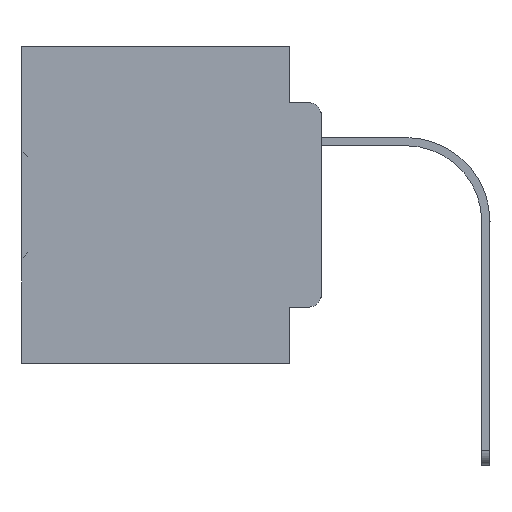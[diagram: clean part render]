
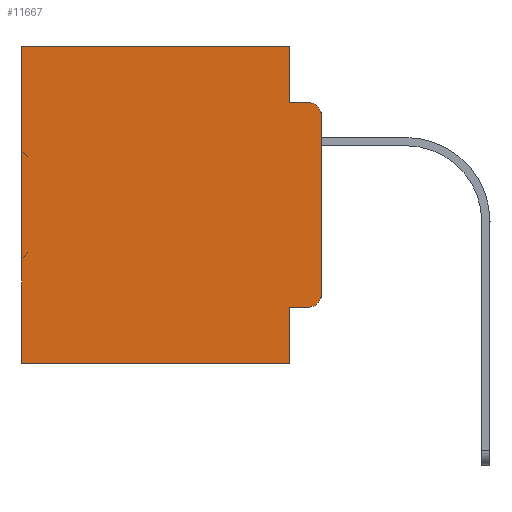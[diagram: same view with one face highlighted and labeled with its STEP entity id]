
A CAD part, left-side view. The second image highlights one B-rep face of the part: STEP entity #11667.
In plain terms, the highlighted planar face has unit normal (-1, 0, 0).
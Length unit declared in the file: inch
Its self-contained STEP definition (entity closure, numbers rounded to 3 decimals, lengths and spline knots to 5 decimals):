
#683 = VERTEX_POINT ( 'NONE', #31722 ) ;
#864 = CARTESIAN_POINT ( 'NONE',  ( 0.298, 0.02, -0.0885 ) ) ;
#2679 = DIRECTION ( 'NONE',  ( 0., 0., -1. ) ) ;
#2912 = DIRECTION ( 'NONE',  ( 0., 0., -1. ) ) ;
#5111 = VERTEX_POINT ( 'NONE', #15395 ) ;
#5186 = ORIENTED_EDGE ( 'NONE', *, *, #19873, .F. ) ;
#6548 = ORIENTED_EDGE ( 'NONE', *, *, #14699, .F. ) ;
#7915 = VECTOR ( 'NONE', #10473, 39.37008 ) ;
#8126 = CARTESIAN_POINT ( 'NONE',  ( 0.298, 0.051, 0. ) ) ;
#8137 = LINE ( 'NONE', #22855, #13507 ) ;
#8353 = LINE ( 'NONE', #14416, #17982 ) ;
#8695 = DIRECTION ( 'NONE',  ( 0., -1., 0. ) ) ;
#9843 = AXIS2_PLACEMENT_3D ( 'NONE', #10184, #36247, #30550 ) ;
#10184 = CARTESIAN_POINT ( 'NONE',  ( 0.298, 0.02, -0.3915 ) ) ;
#10473 = DIRECTION ( 'NONE',  ( 0., 0., -1. ) ) ;
#10853 = CARTESIAN_POINT ( 'NONE',  ( 0.298, 0., 0. ) ) ;
#10874 = ORIENTED_EDGE ( 'NONE', *, *, #19233, .T. ) ;
#11622 = ORIENTED_EDGE ( 'NONE', *, *, #29310, .F. ) ;
#11667 = ADVANCED_FACE ( 'NONE', ( #33702 ), #21825, .F. ) ;
#11980 = EDGE_CURVE ( 'NONE', #24811, #5111, #13129, .T. ) ;
#13129 = LINE ( 'NONE', #30475, #7915 ) ;
#13137 = CARTESIAN_POINT ( 'NONE',  ( 0.298, 0., 0. ) ) ;
#13507 = VECTOR ( 'NONE', #8695, 39.37008 ) ;
#14056 = DIRECTION ( 'NONE',  ( 0., 0., -1. ) ) ;
#14416 = CARTESIAN_POINT ( 'NONE',  ( 0.298, 0.051, -0.4115 ) ) ;
#14699 = EDGE_CURVE ( 'NONE', #35390, #24124, #34506, .T. ) ;
#15132 = VECTOR ( 'NONE', #25929, 39.37008 ) ;
#15395 = CARTESIAN_POINT ( 'NONE',  ( 0.298, 0.051, -0.0885 ) ) ;
#15491 = ORIENTED_EDGE ( 'NONE', *, *, #23393, .T. ) ;
#15737 = AXIS2_PLACEMENT_3D ( 'NONE', #13137, #30297, #16359 ) ;
#15740 = LINE ( 'NONE', #35930, #32511 ) ;
#15836 = EDGE_CURVE ( 'NONE', #32039, #35390, #34621, .T. ) ;
#16308 = VERTEX_POINT ( 'NONE', #29089 ) ;
#16359 = DIRECTION ( 'NONE',  ( 0., 0., -1. ) ) ;
#16947 = CARTESIAN_POINT ( 'NONE',  ( 0.298, 0.02, -0.1085 ) ) ;
#17837 = LINE ( 'NONE', #34813, #15132 ) ;
#17982 = VECTOR ( 'NONE', #25519, 39.37008 ) ;
#18398 = CIRCLE ( 'NONE', #24407, 0.02 ) ;
#19233 = EDGE_CURVE ( 'NONE', #32039, #26867, #8353, .T. ) ;
#19412 = CARTESIAN_POINT ( 'NONE',  ( 0.298, 0.473, -0.5 ) ) ;
#19534 = ORIENTED_EDGE ( 'NONE', *, *, #30064, .T. ) ;
#19577 = VECTOR ( 'NONE', #2912, 39.37008 ) ;
#19873 = EDGE_CURVE ( 'NONE', #16308, #683, #36717, .T. ) ;
#20546 = EDGE_CURVE ( 'NONE', #23524, #24124, #15740, .T. ) ;
#21825 = PLANE ( 'NONE',  #15737 ) ;
#22612 = CARTESIAN_POINT ( 'NONE',  ( 0.298, 0., -0.5 ) ) ;
#22855 = CARTESIAN_POINT ( 'NONE',  ( 0.298, 0.051, -0.0885 ) ) ;
#23393 = EDGE_CURVE ( 'NONE', #24811, #23524, #17837, .T. ) ;
#23473 = CARTESIAN_POINT ( 'NONE',  ( 0.298, 0.051, 0. ) ) ;
#23524 = VERTEX_POINT ( 'NONE', #27598 ) ;
#24039 = ORIENTED_EDGE ( 'NONE', *, *, #11980, .F. ) ;
#24124 = VERTEX_POINT ( 'NONE', #19412 ) ;
#24407 = AXIS2_PLACEMENT_3D ( 'NONE', #16947, #36937, #25774 ) ;
#24553 = CARTESIAN_POINT ( 'NONE',  ( 0.298, 0.051, -0.4115 ) ) ;
#24631 = ORIENTED_EDGE ( 'NONE', *, *, #20546, .T. ) ;
#24811 = VERTEX_POINT ( 'NONE', #8126 ) ;
#25519 = DIRECTION ( 'NONE',  ( 0., -1., 0. ) ) ;
#25774 = DIRECTION ( 'NONE',  ( 0., 0., -1. ) ) ;
#25929 = DIRECTION ( 'NONE',  ( 0., 1., 0. ) ) ;
#26867 = VERTEX_POINT ( 'NONE', #27853 ) ;
#27598 = CARTESIAN_POINT ( 'NONE',  ( 0.298, 0.473, 0. ) ) ;
#27853 = CARTESIAN_POINT ( 'NONE',  ( 0.298, 0.02, -0.4115 ) ) ;
#27895 = ORIENTED_EDGE ( 'NONE', *, *, #28330, .T. ) ;
#28330 = EDGE_CURVE ( 'NONE', #26867, #683, #35167, .T. ) ;
#29089 = CARTESIAN_POINT ( 'NONE',  ( 0.298, 0., -0.1085 ) ) ;
#29310 = EDGE_CURVE ( 'NONE', #5111, #36928, #8137, .T. ) ;
#30064 = EDGE_CURVE ( 'NONE', #16308, #36928, #18398, .T. ) ;
#30297 = DIRECTION ( 'NONE',  ( 1., 0., 0. ) ) ;
#30400 = VECTOR ( 'NONE', #33943, 39.37008 ) ;
#30475 = CARTESIAN_POINT ( 'NONE',  ( 0.298, 0.051, 0. ) ) ;
#30550 = DIRECTION ( 'NONE',  ( 0., 0., -1. ) ) ;
#31722 = CARTESIAN_POINT ( 'NONE',  ( 0.298, 0., -0.3915 ) ) ;
#32039 = VERTEX_POINT ( 'NONE', #24553 ) ;
#32073 = ORIENTED_EDGE ( 'NONE', *, *, #15836, .F. ) ;
#32511 = VECTOR ( 'NONE', #2679, 39.37008 ) ;
#33051 = VECTOR ( 'NONE', #14056, 39.37008 ) ;
#33536 = CARTESIAN_POINT ( 'NONE',  ( 0.298, 0.051, -0.5 ) ) ;
#33702 = FACE_OUTER_BOUND ( 'NONE', #36355, .T. ) ;
#33943 = DIRECTION ( 'NONE',  ( 0., 1., 0. ) ) ;
#34506 = LINE ( 'NONE', #22612, #30400 ) ;
#34621 = LINE ( 'NONE', #23473, #19577 ) ;
#34813 = CARTESIAN_POINT ( 'NONE',  ( 0.298, 0., 0. ) ) ;
#35167 = CIRCLE ( 'NONE', #9843, 0.02 ) ;
#35390 = VERTEX_POINT ( 'NONE', #33536 ) ;
#35930 = CARTESIAN_POINT ( 'NONE',  ( 0.298, 0.473, 0. ) ) ;
#36247 = DIRECTION ( 'NONE',  ( -1., 0., 0. ) ) ;
#36355 = EDGE_LOOP ( 'NONE', ( #5186, #19534, #11622, #24039, #15491, #24631, #6548, #32073, #10874, #27895 ) ) ;
#36717 = LINE ( 'NONE', #10853, #33051 ) ;
#36928 = VERTEX_POINT ( 'NONE', #864 ) ;
#36937 = DIRECTION ( 'NONE',  ( -1., 0., 0. ) ) ;
